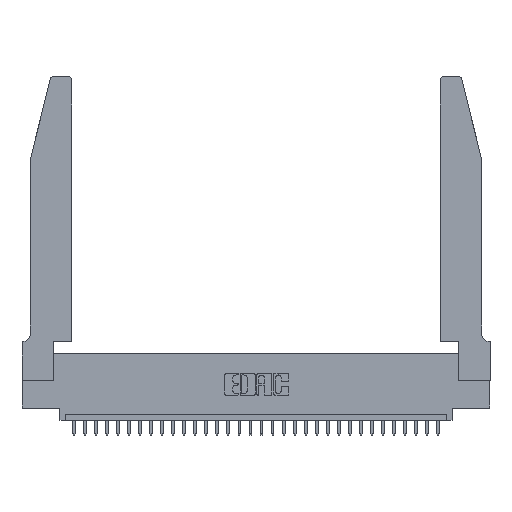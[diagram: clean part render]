
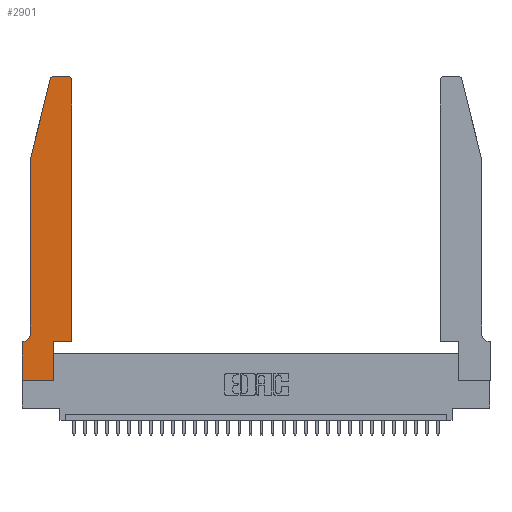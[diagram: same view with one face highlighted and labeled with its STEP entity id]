
A CAD part, top view. The second image highlights one B-rep face of the part: STEP entity #2901.
In plain terms, the highlighted planar face has unit normal (0, 0, 1).
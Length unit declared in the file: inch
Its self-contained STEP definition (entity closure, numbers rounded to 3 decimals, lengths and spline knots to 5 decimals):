
#151 = DIRECTION ( 'NONE',  ( -1., 0., 0. ) ) ;
#169 = CARTESIAN_POINT ( 'NONE',  ( 0.4505, 0.35, 0.37 ) ) ;
#362 = ORIENTED_EDGE ( 'NONE', *, *, #30737, .T. ) ;
#1012 = EDGE_CURVE ( 'NONE', #5103, #16257, #23334, .T. ) ;
#1173 = CIRCLE ( 'NONE', #14442, 0.03 ) ;
#1616 = CARTESIAN_POINT ( 'NONE',  ( 0.25487, 2.72718, 0.37 ) ) ;
#1801 = EDGE_CURVE ( 'NONE', #5407, #27757, #18348, .T. ) ;
#1858 = DIRECTION ( 'NONE',  ( 1., 0., 0. ) ) ;
#2816 = VERTEX_POINT ( 'NONE', #21089 ) ;
#2830 = EDGE_CURVE ( 'NONE', #28686, #19499, #25924, .T. ) ;
#2853 = CARTESIAN_POINT ( 'NONE',  ( 0., 0., 0.37 ) ) ;
#2901 = ADVANCED_FACE ( 'NONE', ( #18663 ), #9269, .T. ) ;
#3227 = CARTESIAN_POINT ( 'NONE',  ( 0.2865, 0.35, 0.37 ) ) ;
#3247 = CARTESIAN_POINT ( 'NONE',  ( 0.4205, 2.72, 0.37 ) ) ;
#4095 = LINE ( 'NONE', #15665, #6751 ) ;
#4356 = VECTOR ( 'NONE', #12368, 39.37008 ) ;
#4736 = EDGE_CURVE ( 'NONE', #27757, #13698, #4095, .T. ) ;
#4941 = LINE ( 'NONE', #3227, #27422 ) ;
#5037 = CARTESIAN_POINT ( 'NONE',  ( 0.2605, 2.75, 0.37 ) ) ;
#5103 = VERTEX_POINT ( 'NONE', #26951 ) ;
#5230 = CARTESIAN_POINT ( 'NONE',  ( 0.2865, 0.35, 0.37 ) ) ;
#5328 = ORIENTED_EDGE ( 'NONE', *, *, #1801, .T. ) ;
#5407 = VERTEX_POINT ( 'NONE', #6081 ) ;
#5463 = CARTESIAN_POINT ( 'NONE',  ( 0.4505, 0.35, 0.37 ) ) ;
#6081 = CARTESIAN_POINT ( 'NONE',  ( 0.0055, 0.35, 0.37 ) ) ;
#6477 = ORIENTED_EDGE ( 'NONE', *, *, #4736, .T. ) ;
#6721 = ORIENTED_EDGE ( 'NONE', *, *, #24391, .T. ) ;
#6751 = VECTOR ( 'NONE', #25179, 39.37008 ) ;
#7477 = ORIENTED_EDGE ( 'NONE', *, *, #9553, .T. ) ;
#7529 = DIRECTION ( 'NONE',  ( 1., 0., 0. ) ) ;
#7779 = AXIS2_PLACEMENT_3D ( 'NONE', #11483, #28576, #1858 ) ;
#8914 = CARTESIAN_POINT ( 'NONE',  ( 0.284, 2.72, 0.37 ) ) ;
#9269 = PLANE ( 'NONE',  #7779 ) ;
#9553 = EDGE_CURVE ( 'NONE', #13698, #14395, #18147, .T. ) ;
#9605 = VECTOR ( 'NONE', #19143, 39.37008 ) ;
#9785 = CARTESIAN_POINT ( 'NONE',  ( 0.0755, 2., 0.37 ) ) ;
#9969 = DIRECTION ( 'NONE',  ( 0., -1., 0. ) ) ;
#10890 = EDGE_LOOP ( 'NONE', ( #17240, #22199, #362, #23164, #26545, #5328, #6477, #7477, #24063, #21693, #27447, #6721 ) ) ;
#10942 = CARTESIAN_POINT ( 'NONE',  ( 0., 0., 0.37 ) ) ;
#10978 = CARTESIAN_POINT ( 'NONE',  ( 0., 0.35, 0.37 ) ) ;
#11483 = CARTESIAN_POINT ( 'NONE',  ( 0., 0.35, 0.37 ) ) ;
#11668 = VECTOR ( 'NONE', #7529, 39.37008 ) ;
#11829 = EDGE_CURVE ( 'NONE', #19499, #11874, #22248, .T. ) ;
#11874 = VERTEX_POINT ( 'NONE', #29979 ) ;
#12368 = DIRECTION ( 'NONE',  ( 0., 1., 0. ) ) ;
#12487 = DIRECTION ( 'NONE',  ( 1., 0., 0. ) ) ;
#13065 = CIRCLE ( 'NONE', #13082, 0.07 ) ;
#13082 = AXIS2_PLACEMENT_3D ( 'NONE', #16491, #19047, #31451 ) ;
#13615 = VERTEX_POINT ( 'NONE', #1616 ) ;
#13698 = VERTEX_POINT ( 'NONE', #10942 ) ;
#14048 = VECTOR ( 'NONE', #24729, 39.37008 ) ;
#14395 = VERTEX_POINT ( 'NONE', #29158 ) ;
#14442 = AXIS2_PLACEMENT_3D ( 'NONE', #3247, #20265, #12487 ) ;
#14901 = CARTESIAN_POINT ( 'NONE',  ( 0.4205, 2.75, 0.37 ) ) ;
#15665 = CARTESIAN_POINT ( 'NONE',  ( 0., 0., 0.37 ) ) ;
#15774 = DIRECTION ( 'NONE',  ( 1., 0., 0. ) ) ;
#16257 = VERTEX_POINT ( 'NONE', #29499 ) ;
#16491 = CARTESIAN_POINT ( 'NONE',  ( 0.0055, 0.42, 0.37 ) ) ;
#16865 = VECTOR ( 'NONE', #9969, 39.37008 ) ;
#16997 = DIRECTION ( 'NONE',  ( 0., 0., 1. ) ) ;
#17159 = VECTOR ( 'NONE', #15774, 39.37008 ) ;
#17222 = CARTESIAN_POINT ( 'NONE',  ( 0.0755, 2., 0.37 ) ) ;
#17240 = ORIENTED_EDGE ( 'NONE', *, *, #19345, .T. ) ;
#18147 = LINE ( 'NONE', #2853, #11668 ) ;
#18348 = LINE ( 'NONE', #23974, #9605 ) ;
#18621 = LINE ( 'NONE', #9785, #14048 ) ;
#18663 = FACE_OUTER_BOUND ( 'NONE', #10890, .T. ) ;
#19047 = DIRECTION ( 'NONE',  ( 0., 0., -1. ) ) ;
#19143 = DIRECTION ( 'NONE',  ( -1., 0., 0. ) ) ;
#19345 = EDGE_CURVE ( 'NONE', #28698, #2816, #26924, .T. ) ;
#19499 = VERTEX_POINT ( 'NONE', #5463 ) ;
#20265 = DIRECTION ( 'NONE',  ( 0., 0., 1. ) ) ;
#20443 = VECTOR ( 'NONE', #151, 39.37008 ) ;
#21089 = CARTESIAN_POINT ( 'NONE',  ( 0.284, 2.75, 0.37 ) ) ;
#21693 = ORIENTED_EDGE ( 'NONE', *, *, #2830, .T. ) ;
#22199 = ORIENTED_EDGE ( 'NONE', *, *, #27209, .T. ) ;
#22248 = LINE ( 'NONE', #169, #4356 ) ;
#23164 = ORIENTED_EDGE ( 'NONE', *, *, #1012, .T. ) ;
#23334 = LINE ( 'NONE', #17222, #16865 ) ;
#23852 = CIRCLE ( 'NONE', #30248, 0.03 ) ;
#23974 = CARTESIAN_POINT ( 'NONE',  ( 0.0755, 0.35, 0.37 ) ) ;
#24063 = ORIENTED_EDGE ( 'NONE', *, *, #24976, .T. ) ;
#24391 = EDGE_CURVE ( 'NONE', #11874, #28698, #1173, .T. ) ;
#24729 = DIRECTION ( 'NONE',  ( -0.239, -0.971, 0. ) ) ;
#24976 = EDGE_CURVE ( 'NONE', #14395, #28686, #4941, .T. ) ;
#25179 = DIRECTION ( 'NONE',  ( 0., -1., 0. ) ) ;
#25924 = LINE ( 'NONE', #27927, #17159 ) ;
#26545 = ORIENTED_EDGE ( 'NONE', *, *, #28520, .T. ) ;
#26924 = LINE ( 'NONE', #5037, #20443 ) ;
#26951 = CARTESIAN_POINT ( 'NONE',  ( 0.0755, 2., 0.37 ) ) ;
#27209 = EDGE_CURVE ( 'NONE', #2816, #13615, #23852, .T. ) ;
#27422 = VECTOR ( 'NONE', #27496, 39.37008 ) ;
#27447 = ORIENTED_EDGE ( 'NONE', *, *, #11829, .T. ) ;
#27496 = DIRECTION ( 'NONE',  ( 0., 1., 0. ) ) ;
#27757 = VERTEX_POINT ( 'NONE', #10978 ) ;
#27927 = CARTESIAN_POINT ( 'NONE',  ( 0.4505, 0.35, 0.37 ) ) ;
#28520 = EDGE_CURVE ( 'NONE', #16257, #5407, #13065, .T. ) ;
#28576 = DIRECTION ( 'NONE',  ( 0., 0., 1. ) ) ;
#28686 = VERTEX_POINT ( 'NONE', #5230 ) ;
#28698 = VERTEX_POINT ( 'NONE', #14901 ) ;
#29158 = CARTESIAN_POINT ( 'NONE',  ( 0.2865, 0., 0.37 ) ) ;
#29168 = DIRECTION ( 'NONE',  ( 1., 0., 0. ) ) ;
#29499 = CARTESIAN_POINT ( 'NONE',  ( 0.0755, 0.42, 0.37 ) ) ;
#29979 = CARTESIAN_POINT ( 'NONE',  ( 0.4505, 2.72, 0.37 ) ) ;
#30248 = AXIS2_PLACEMENT_3D ( 'NONE', #8914, #16997, #29168 ) ;
#30737 = EDGE_CURVE ( 'NONE', #13615, #5103, #18621, .T. ) ;
#31451 = DIRECTION ( 'NONE',  ( -1., 0., 0. ) ) ;
